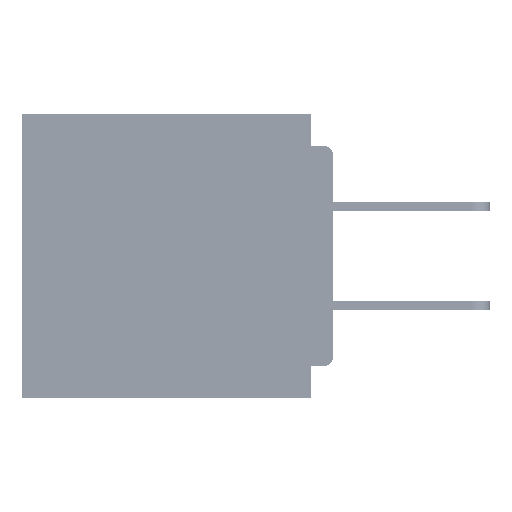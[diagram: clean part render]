
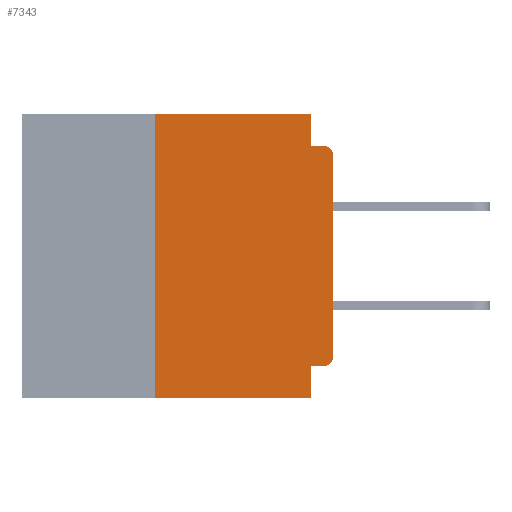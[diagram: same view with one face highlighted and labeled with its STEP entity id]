
A CAD part, left-side view. The second image highlights one B-rep face of the part: STEP entity #7343.
In plain terms, the highlighted planar face has unit normal (-1, 0, 0).
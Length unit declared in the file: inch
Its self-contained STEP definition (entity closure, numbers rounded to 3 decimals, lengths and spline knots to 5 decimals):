
#458 = CARTESIAN_POINT ( 'NONE',  ( 0., 0.015, -0.355 ) ) ;
#775 = CARTESIAN_POINT ( 'NONE',  ( 0., 0.25, -0.4 ) ) ;
#1613 = ORIENTED_EDGE ( 'NONE', *, *, #7714, .T. ) ;
#2187 = CARTESIAN_POINT ( 'NONE',  ( 0., 0.015, -0.34 ) ) ;
#2507 = DIRECTION ( 'NONE',  ( 0., 0., 1. ) ) ;
#2562 = VERTEX_POINT ( 'NONE', #458 ) ;
#2779 = DIRECTION ( 'NONE',  ( 0., 0., -1. ) ) ;
#3306 = LINE ( 'NONE', #51865, #55924 ) ;
#3314 = ORIENTED_EDGE ( 'NONE', *, *, #15850, .F. ) ;
#4289 = DIRECTION ( 'NONE',  ( 0., 0., -1. ) ) ;
#4687 = ORIENTED_EDGE ( 'NONE', *, *, #14269, .T. ) ;
#5582 = VERTEX_POINT ( 'NONE', #25305 ) ;
#7341 = DIRECTION ( 'NONE',  ( 0., 0., -1. ) ) ;
#7343 = ADVANCED_FACE ( 'NONE', ( #41877 ), #60146, .F. ) ;
#7714 = EDGE_CURVE ( 'NONE', #2562, #39237, #58385, .T. ) ;
#7767 = DIRECTION ( 'NONE',  ( 0., 0., -1. ) ) ;
#7861 = DIRECTION ( 'NONE',  ( 0., 1., 0. ) ) ;
#10394 = CARTESIAN_POINT ( 'NONE',  ( 0., 0.031, 0. ) ) ;
#11072 = CARTESIAN_POINT ( 'NONE',  ( 0., 0., -0.06 ) ) ;
#11742 = LINE ( 'NONE', #48367, #37392 ) ;
#11969 = CARTESIAN_POINT ( 'NONE',  ( 0., 0., -0.34 ) ) ;
#14239 = DIRECTION ( 'NONE',  ( 0., -1., 0. ) ) ;
#14240 = AXIS2_PLACEMENT_3D ( 'NONE', #29771, #34957, #4289 ) ;
#14269 = EDGE_CURVE ( 'NONE', #29281, #21291, #45159, .T. ) ;
#15850 = EDGE_CURVE ( 'NONE', #56074, #37759, #3306, .T. ) ;
#18654 = VERTEX_POINT ( 'NONE', #45450 ) ;
#18825 = VECTOR ( 'NONE', #7861, 39.37008 ) ;
#21040 = EDGE_CURVE ( 'NONE', #65576, #18654, #60458, .T. ) ;
#21291 = VERTEX_POINT ( 'NONE', #61413 ) ;
#21561 = VECTOR ( 'NONE', #59217, 39.37008 ) ;
#23226 = VECTOR ( 'NONE', #2507, 39.37008 ) ;
#23276 = AXIS2_PLACEMENT_3D ( 'NONE', #2187, #38026, #7341 ) ;
#23738 = CARTESIAN_POINT ( 'NONE',  ( 0., 0., -0.045 ) ) ;
#25305 = CARTESIAN_POINT ( 'NONE',  ( 0., 0.031, -0.355 ) ) ;
#26001 = ORIENTED_EDGE ( 'NONE', *, *, #61797, .F. ) ;
#27208 = EDGE_CURVE ( 'NONE', #2562, #5582, #32436, .T. ) ;
#28014 = CARTESIAN_POINT ( 'NONE',  ( 0., 0., 0. ) ) ;
#29171 = DIRECTION ( 'NONE',  ( 0., 0., -1. ) ) ;
#29281 = VERTEX_POINT ( 'NONE', #35186 ) ;
#29431 = CARTESIAN_POINT ( 'NONE',  ( 0., 0.437, -0.4 ) ) ;
#29771 = CARTESIAN_POINT ( 'NONE',  ( 0., 0.437, 0. ) ) ;
#30011 = VECTOR ( 'NONE', #14239, 39.37008 ) ;
#30111 = CARTESIAN_POINT ( 'NONE',  ( 0., 0.25, 0. ) ) ;
#30926 = EDGE_CURVE ( 'NONE', #39237, #42990, #35225, .T. ) ;
#31479 = EDGE_LOOP ( 'NONE', ( #54737, #42898, #61081, #35782, #3314, #26001, #4687, #48573, #31897, #1613 ) ) ;
#31897 = ORIENTED_EDGE ( 'NONE', *, *, #27208, .F. ) ;
#32436 = LINE ( 'NONE', #38516, #18825 ) ;
#33454 = DIRECTION ( 'NONE',  ( -1., 0., 0. ) ) ;
#34957 = DIRECTION ( 'NONE',  ( 1., 0., 0. ) ) ;
#35186 = CARTESIAN_POINT ( 'NONE',  ( 0., 0.25, -0.4 ) ) ;
#35225 = LINE ( 'NONE', #28014, #23226 ) ;
#35782 = ORIENTED_EDGE ( 'NONE', *, *, #53570, .F. ) ;
#35898 = AXIS2_PLACEMENT_3D ( 'NONE', #63753, #33454, #2779 ) ;
#36634 = DIRECTION ( 'NONE',  ( 0., 0., 1. ) ) ;
#36837 = DIRECTION ( 'NONE',  ( 0., -1., 0. ) ) ;
#37392 = VECTOR ( 'NONE', #7767, 39.37008 ) ;
#37759 = VERTEX_POINT ( 'NONE', #10394 ) ;
#38026 = DIRECTION ( 'NONE',  ( -1., 0., 0. ) ) ;
#38516 = CARTESIAN_POINT ( 'NONE',  ( 0., 0., -0.355 ) ) ;
#39237 = VERTEX_POINT ( 'NONE', #11969 ) ;
#41877 = FACE_OUTER_BOUND ( 'NONE', #31479, .T. ) ;
#42898 = ORIENTED_EDGE ( 'NONE', *, *, #47146, .T. ) ;
#42990 = VERTEX_POINT ( 'NONE', #11072 ) ;
#45159 = LINE ( 'NONE', #29431, #30011 ) ;
#45450 = CARTESIAN_POINT ( 'NONE',  ( 0., 0.015, -0.045 ) ) ;
#47146 = EDGE_CURVE ( 'NONE', #42990, #18654, #59764, .T. ) ;
#48367 = CARTESIAN_POINT ( 'NONE',  ( 0., 0.031, 0. ) ) ;
#48421 = LINE ( 'NONE', #775, #61881 ) ;
#48573 = ORIENTED_EDGE ( 'NONE', *, *, #62128, .F. ) ;
#51865 = CARTESIAN_POINT ( 'NONE',  ( 0., 0.437, 0. ) ) ;
#53143 = LINE ( 'NONE', #54486, #64986 ) ;
#53189 = CARTESIAN_POINT ( 'NONE',  ( 0., 0.031, -0.045 ) ) ;
#53570 = EDGE_CURVE ( 'NONE', #37759, #65576, #11742, .T. ) ;
#54486 = CARTESIAN_POINT ( 'NONE',  ( 0., 0.031, -0.4 ) ) ;
#54737 = ORIENTED_EDGE ( 'NONE', *, *, #30926, .T. ) ;
#55924 = VECTOR ( 'NONE', #36837, 39.37008 ) ;
#56074 = VERTEX_POINT ( 'NONE', #30111 ) ;
#58385 = CIRCLE ( 'NONE', #23276, 0.015 ) ;
#59217 = DIRECTION ( 'NONE',  ( 0., -1., 0. ) ) ;
#59764 = CIRCLE ( 'NONE', #35898, 0.015 ) ;
#60146 = PLANE ( 'NONE',  #14240 ) ;
#60458 = LINE ( 'NONE', #23738, #21561 ) ;
#61081 = ORIENTED_EDGE ( 'NONE', *, *, #21040, .F. ) ;
#61413 = CARTESIAN_POINT ( 'NONE',  ( 0., 0.031, -0.4 ) ) ;
#61797 = EDGE_CURVE ( 'NONE', #29281, #56074, #48421, .T. ) ;
#61881 = VECTOR ( 'NONE', #36634, 39.37008 ) ;
#62128 = EDGE_CURVE ( 'NONE', #5582, #21291, #53143, .T. ) ;
#63753 = CARTESIAN_POINT ( 'NONE',  ( 0., 0.015, -0.06 ) ) ;
#64986 = VECTOR ( 'NONE', #29171, 39.37008 ) ;
#65576 = VERTEX_POINT ( 'NONE', #53189 ) ;
